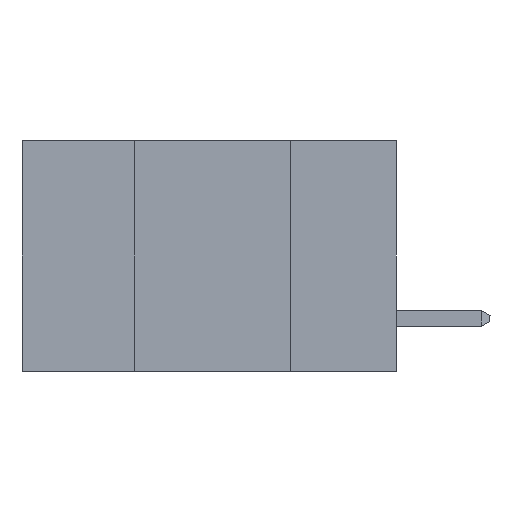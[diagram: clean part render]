
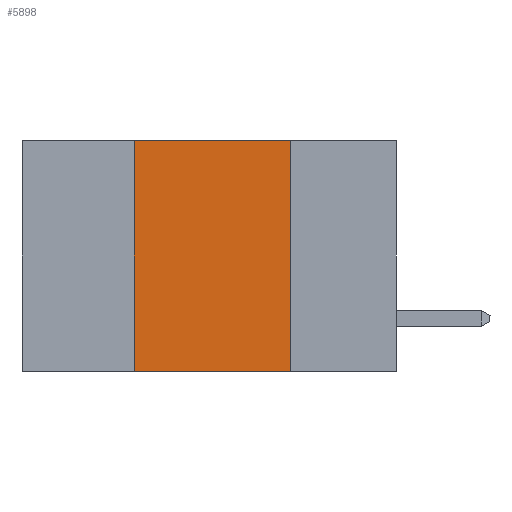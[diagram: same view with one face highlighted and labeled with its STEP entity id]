
A CAD part, left-side view. The second image highlights one B-rep face of the part: STEP entity #5898.
In plain terms, the highlighted planar face has unit normal (-1, 0, 0).
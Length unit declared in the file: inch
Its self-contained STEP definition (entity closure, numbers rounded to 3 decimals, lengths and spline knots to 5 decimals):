
#56 = DIRECTION ( 'NONE',  ( 0., -1., 0. ) ) ;
#107 = VERTEX_POINT ( 'NONE', #8278 ) ;
#1212 = VERTEX_POINT ( 'NONE', #3641 ) ;
#1406 = CARTESIAN_POINT ( 'NONE',  ( 0., 0.6, -0.37 ) ) ;
#1447 = CARTESIAN_POINT ( 'NONE',  ( 0., 0.17, -0.37 ) ) ;
#1460 = DIRECTION ( 'NONE',  ( 0., 0., 1. ) ) ;
#1631 = VECTOR ( 'NONE', #7819, 39.37008 ) ;
#2470 = EDGE_CURVE ( 'NONE', #1212, #4487, #8067, .T. ) ;
#2489 = CARTESIAN_POINT ( 'NONE',  ( 0., 0.6, 0. ) ) ;
#2691 = VECTOR ( 'NONE', #1460, 39.37008 ) ;
#2789 = VECTOR ( 'NONE', #56, 39.37008 ) ;
#2895 = LINE ( 'NONE', #5189, #2691 ) ;
#2972 = ORIENTED_EDGE ( 'NONE', *, *, #2470, .F. ) ;
#3251 = DIRECTION ( 'NONE',  ( 0., 0., -1. ) ) ;
#3641 = CARTESIAN_POINT ( 'NONE',  ( 0., 0.42, 0. ) ) ;
#3944 = EDGE_LOOP ( 'NONE', ( #4097, #2972, #4207, #5396 ) ) ;
#4047 = PLANE ( 'NONE',  #8924 ) ;
#4097 = ORIENTED_EDGE ( 'NONE', *, *, #7812, .F. ) ;
#4207 = ORIENTED_EDGE ( 'NONE', *, *, #4821, .F. ) ;
#4487 = VERTEX_POINT ( 'NONE', #8920 ) ;
#4625 = FACE_OUTER_BOUND ( 'NONE', #3944, .T. ) ;
#4821 = EDGE_CURVE ( 'NONE', #6859, #1212, #2895, .T. ) ;
#5189 = CARTESIAN_POINT ( 'NONE',  ( 0., 0.42, -0.37 ) ) ;
#5396 = ORIENTED_EDGE ( 'NONE', *, *, #7367, .T. ) ;
#5616 = LINE ( 'NONE', #1406, #1631 ) ;
#5898 = ADVANCED_FACE ( 'NONE', ( #4625 ), #4047, .F. ) ;
#6859 = VERTEX_POINT ( 'NONE', #8442 ) ;
#7180 = DIRECTION ( 'NONE',  ( 0., 0., -1. ) ) ;
#7367 = EDGE_CURVE ( 'NONE', #6859, #107, #5616, .T. ) ;
#7433 = VECTOR ( 'NONE', #7180, 39.37008 ) ;
#7589 = DIRECTION ( 'NONE',  ( 1., 0., 0. ) ) ;
#7812 = EDGE_CURVE ( 'NONE', #4487, #107, #9231, .T. ) ;
#7819 = DIRECTION ( 'NONE',  ( 0., -1., 0. ) ) ;
#8067 = LINE ( 'NONE', #8817, #2789 ) ;
#8278 = CARTESIAN_POINT ( 'NONE',  ( 0., 0.17, -0.37 ) ) ;
#8442 = CARTESIAN_POINT ( 'NONE',  ( 0., 0.42, -0.37 ) ) ;
#8817 = CARTESIAN_POINT ( 'NONE',  ( 0., 0.6, 0. ) ) ;
#8920 = CARTESIAN_POINT ( 'NONE',  ( 0., 0.17, 0. ) ) ;
#8924 = AXIS2_PLACEMENT_3D ( 'NONE', #2489, #7589, #3251 ) ;
#9231 = LINE ( 'NONE', #1447, #7433 ) ;
